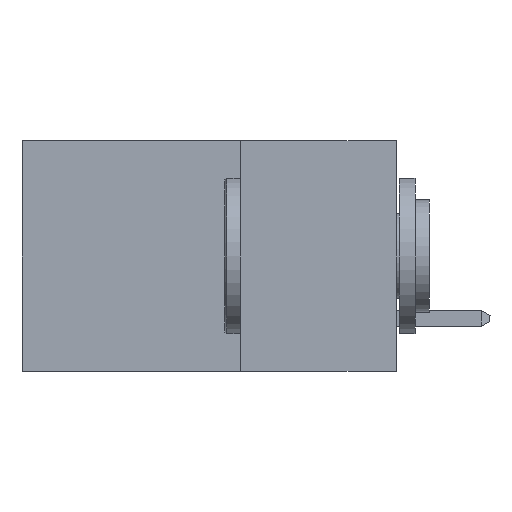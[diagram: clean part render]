
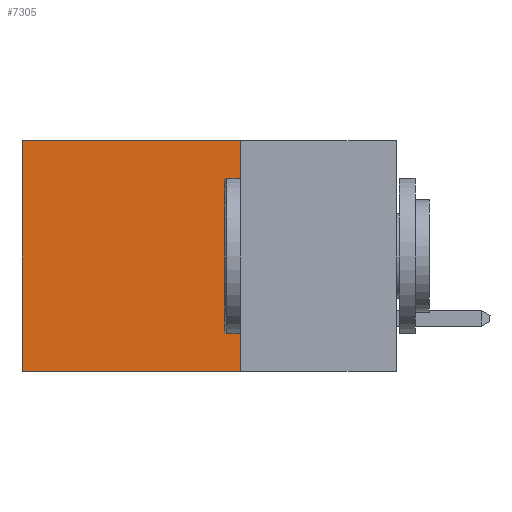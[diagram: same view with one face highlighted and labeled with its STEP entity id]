
A CAD part, left-side view. The second image highlights one B-rep face of the part: STEP entity #7305.
In plain terms, the highlighted planar face has unit normal (-1, 0, 0).
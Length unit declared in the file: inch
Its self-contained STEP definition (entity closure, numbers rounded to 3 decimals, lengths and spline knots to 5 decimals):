
#291 = DIRECTION ( 'NONE',  ( 0., 0., -1. ) ) ;
#628 = EDGE_CURVE ( 'NONE', #2729, #10319, #5998, .T. ) ;
#1383 = DIRECTION ( 'NONE',  ( 1., 0., 0. ) ) ;
#1656 = EDGE_CURVE ( 'NONE', #6875, #10319, #8981, .T. ) ;
#2027 = ORIENTED_EDGE ( 'NONE', *, *, #1656, .F. ) ;
#2063 = CARTESIAN_POINT ( 'NONE',  ( 0.2615, 0.6, -0.37 ) ) ;
#2265 = AXIS2_PLACEMENT_3D ( 'NONE', #3384, #1383, #8271 ) ;
#2596 = EDGE_CURVE ( 'NONE', #6822, #2729, #12119, .T. ) ;
#2729 = VERTEX_POINT ( 'NONE', #11665 ) ;
#3343 = VECTOR ( 'NONE', #9219, 39.37008 ) ;
#3384 = CARTESIAN_POINT ( 'NONE',  ( 0.2615, 0.25, -0.37 ) ) ;
#3408 = CARTESIAN_POINT ( 'NONE',  ( 0.2615, 0.6, -0.37 ) ) ;
#5347 = ORIENTED_EDGE ( 'NONE', *, *, #2596, .T. ) ;
#5422 = CARTESIAN_POINT ( 'NONE',  ( 0.2615, 0.25, -0.37 ) ) ;
#5433 = FACE_OUTER_BOUND ( 'NONE', #5707, .T. ) ;
#5707 = EDGE_LOOP ( 'NONE', ( #7906, #2027, #10570, #5347 ) ) ;
#5998 = LINE ( 'NONE', #3408, #3343 ) ;
#6822 = VERTEX_POINT ( 'NONE', #10375 ) ;
#6875 = VERTEX_POINT ( 'NONE', #9550 ) ;
#6879 = DIRECTION ( 'NONE',  ( 0., 1., 0. ) ) ;
#7148 = CARTESIAN_POINT ( 'NONE',  ( 0.2615, 0.25, 0. ) ) ;
#7274 = EDGE_CURVE ( 'NONE', #6822, #6875, #10279, .T. ) ;
#7305 = ADVANCED_FACE ( 'NONE', ( #5433 ), #11830, .F. ) ;
#7905 = VECTOR ( 'NONE', #291, 39.37008 ) ;
#7906 = ORIENTED_EDGE ( 'NONE', *, *, #628, .T. ) ;
#8271 = DIRECTION ( 'NONE',  ( 0., 0., -1. ) ) ;
#8691 = VECTOR ( 'NONE', #11750, 39.37008 ) ;
#8981 = LINE ( 'NONE', #12201, #8691 ) ;
#9219 = DIRECTION ( 'NONE',  ( 0., 0., -1. ) ) ;
#9550 = CARTESIAN_POINT ( 'NONE',  ( 0.2615, 0.25, -0.37 ) ) ;
#9756 = VECTOR ( 'NONE', #6879, 39.37008 ) ;
#10279 = LINE ( 'NONE', #5422, #7905 ) ;
#10319 = VERTEX_POINT ( 'NONE', #2063 ) ;
#10375 = CARTESIAN_POINT ( 'NONE',  ( 0.2615, 0.25, 0. ) ) ;
#10570 = ORIENTED_EDGE ( 'NONE', *, *, #7274, .F. ) ;
#11665 = CARTESIAN_POINT ( 'NONE',  ( 0.2615, 0.6, 0. ) ) ;
#11750 = DIRECTION ( 'NONE',  ( 0., 1., 0. ) ) ;
#11830 = PLANE ( 'NONE',  #2265 ) ;
#12119 = LINE ( 'NONE', #7148, #9756 ) ;
#12201 = CARTESIAN_POINT ( 'NONE',  ( 0.2615, 0.25, -0.37 ) ) ;
